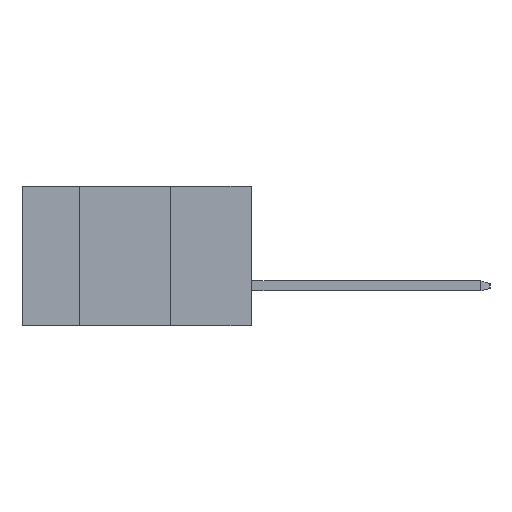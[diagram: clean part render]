
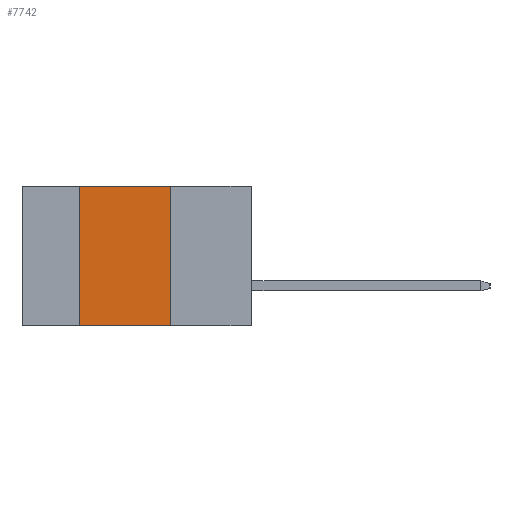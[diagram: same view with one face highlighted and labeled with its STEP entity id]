
A CAD part, left-side view. The second image highlights one B-rep face of the part: STEP entity #7742.
In plain terms, the highlighted planar face has unit normal (-1, 0, 0).
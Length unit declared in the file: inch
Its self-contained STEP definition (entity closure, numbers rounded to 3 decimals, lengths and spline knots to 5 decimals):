
#226 = FACE_OUTER_BOUND ( 'NONE', #6437, .T. ) ;
#736 = CARTESIAN_POINT ( 'NONE',  ( 0., 0.254, -0.437 ) ) ;
#924 = LINE ( 'NONE', #8764, #8176 ) ;
#1851 = DIRECTION ( 'NONE',  ( 0., 0., 1. ) ) ;
#1943 = VERTEX_POINT ( 'NONE', #8120 ) ;
#2434 = ORIENTED_EDGE ( 'NONE', *, *, #7649, .F. ) ;
#2492 = DIRECTION ( 'NONE',  ( 0., 0., -1. ) ) ;
#2951 = DIRECTION ( 'NONE',  ( 0., 0., -1. ) ) ;
#3058 = EDGE_CURVE ( 'NONE', #1943, #10049, #7894, .T. ) ;
#3086 = LINE ( 'NONE', #8367, #10917 ) ;
#3346 = CARTESIAN_POINT ( 'NONE',  ( 0., 0.254, -0.437 ) ) ;
#3760 = CARTESIAN_POINT ( 'NONE',  ( 0., 0.72, -0.437 ) ) ;
#4824 = EDGE_CURVE ( 'NONE', #5794, #1943, #3086, .T. ) ;
#4874 = ORIENTED_EDGE ( 'NONE', *, *, #7775, .T. ) ;
#4993 = VECTOR ( 'NONE', #5504, 39.37008 ) ;
#5113 = ORIENTED_EDGE ( 'NONE', *, *, #3058, .F. ) ;
#5504 = DIRECTION ( 'NONE',  ( 0., -1., 0. ) ) ;
#5616 = CARTESIAN_POINT ( 'NONE',  ( 0., 0.72, 0. ) ) ;
#5666 = DIRECTION ( 'NONE',  ( 1., 0., 0. ) ) ;
#5794 = VERTEX_POINT ( 'NONE', #10238 ) ;
#6437 = EDGE_LOOP ( 'NONE', ( #5113, #9920, #2434, #4874 ) ) ;
#6484 = AXIS2_PLACEMENT_3D ( 'NONE', #5616, #5666, #2951 ) ;
#7451 = DIRECTION ( 'NONE',  ( 0., -1., 0. ) ) ;
#7649 = EDGE_CURVE ( 'NONE', #10789, #5794, #924, .T. ) ;
#7742 = ADVANCED_FACE ( 'NONE', ( #226 ), #8183, .F. ) ;
#7775 = EDGE_CURVE ( 'NONE', #10789, #10049, #8237, .T. ) ;
#7894 = LINE ( 'NONE', #3346, #10202 ) ;
#8120 = CARTESIAN_POINT ( 'NONE',  ( 0., 0.254, 0. ) ) ;
#8176 = VECTOR ( 'NONE', #1851, 39.37008 ) ;
#8183 = PLANE ( 'NONE',  #6484 ) ;
#8237 = LINE ( 'NONE', #3760, #4993 ) ;
#8245 = CARTESIAN_POINT ( 'NONE',  ( 0., 0.54, -0.437 ) ) ;
#8367 = CARTESIAN_POINT ( 'NONE',  ( 0., 0.72, 0. ) ) ;
#8764 = CARTESIAN_POINT ( 'NONE',  ( 0., 0.54, -0.437 ) ) ;
#9920 = ORIENTED_EDGE ( 'NONE', *, *, #4824, .F. ) ;
#10049 = VERTEX_POINT ( 'NONE', #736 ) ;
#10202 = VECTOR ( 'NONE', #2492, 39.37008 ) ;
#10238 = CARTESIAN_POINT ( 'NONE',  ( 0., 0.54, 0. ) ) ;
#10789 = VERTEX_POINT ( 'NONE', #8245 ) ;
#10917 = VECTOR ( 'NONE', #7451, 39.37008 ) ;
